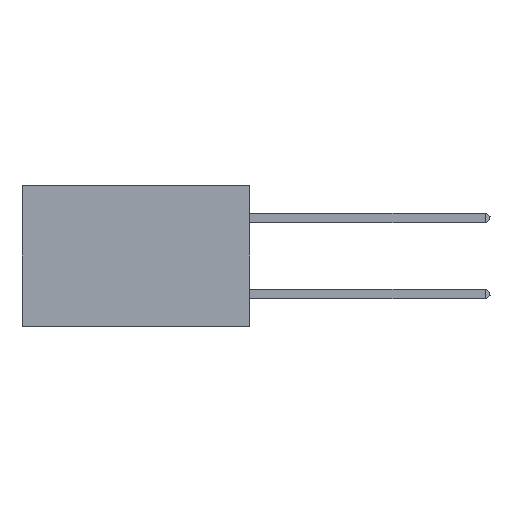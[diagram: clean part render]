
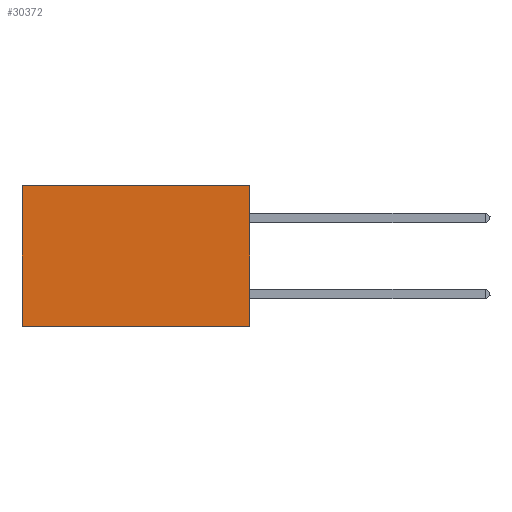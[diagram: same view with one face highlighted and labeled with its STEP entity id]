
A CAD part, left-side view. The second image highlights one B-rep face of the part: STEP entity #30372.
In plain terms, the highlighted planar face has unit normal (-1, 0, 0).
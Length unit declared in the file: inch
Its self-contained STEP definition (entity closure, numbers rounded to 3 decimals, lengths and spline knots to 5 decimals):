
#605 = DIRECTION ( 'NONE',  ( 0., 1., 0. ) ) ;
#3188 = ORIENTED_EDGE ( 'NONE', *, *, #27083, .F. ) ;
#3413 = DIRECTION ( 'NONE',  ( 0., 0., -1. ) ) ;
#5521 = DIRECTION ( 'NONE',  ( 0., 0., -1. ) ) ;
#5573 = ORIENTED_EDGE ( 'NONE', *, *, #12115, .F. ) ;
#7573 = AXIS2_PLACEMENT_3D ( 'NONE', #19884, #30374, #27205 ) ;
#8574 = EDGE_CURVE ( 'NONE', #14365, #45334, #22347, .T. ) ;
#9254 = CARTESIAN_POINT ( 'NONE',  ( 0.2875, 0.6, 0. ) ) ;
#12115 = EDGE_CURVE ( 'NONE', #43734, #46641, #36750, .T. ) ;
#14365 = VERTEX_POINT ( 'NONE', #9254 ) ;
#14827 = CARTESIAN_POINT ( 'NONE',  ( 0.2875, 0., -0.37 ) ) ;
#17012 = LINE ( 'NONE', #34792, #41972 ) ;
#19884 = CARTESIAN_POINT ( 'NONE',  ( 0.2875, 0., 0. ) ) ;
#21505 = EDGE_CURVE ( 'NONE', #43734, #14365, #17012, .T. ) ;
#22347 = LINE ( 'NONE', #27284, #35377 ) ;
#22692 = CARTESIAN_POINT ( 'NONE',  ( 0.2875, 0., -0.37 ) ) ;
#22699 = EDGE_LOOP ( 'NONE', ( #24024, #3188, #5573, #31889 ) ) ;
#23482 = LINE ( 'NONE', #22692, #39367 ) ;
#24024 = ORIENTED_EDGE ( 'NONE', *, *, #8574, .T. ) ;
#27083 = EDGE_CURVE ( 'NONE', #46641, #45334, #23482, .T. ) ;
#27205 = DIRECTION ( 'NONE',  ( 0., 0., -1. ) ) ;
#27284 = CARTESIAN_POINT ( 'NONE',  ( 0.2875, 0.6, 0. ) ) ;
#30372 = ADVANCED_FACE ( 'NONE', ( #33926 ), #34445, .F. ) ;
#30374 = DIRECTION ( 'NONE',  ( 1., 0., 0. ) ) ;
#30517 = CARTESIAN_POINT ( 'NONE',  ( 0.2875, 0., 0. ) ) ;
#31889 = ORIENTED_EDGE ( 'NONE', *, *, #21505, .T. ) ;
#32306 = CARTESIAN_POINT ( 'NONE',  ( 0.2875, 0., 0. ) ) ;
#33334 = VECTOR ( 'NONE', #3413, 39.37008 ) ;
#33926 = FACE_OUTER_BOUND ( 'NONE', #22699, .T. ) ;
#34445 = PLANE ( 'NONE',  #7573 ) ;
#34792 = CARTESIAN_POINT ( 'NONE',  ( 0.2875, 0., 0. ) ) ;
#35377 = VECTOR ( 'NONE', #5521, 39.37008 ) ;
#36750 = LINE ( 'NONE', #32306, #33334 ) ;
#39367 = VECTOR ( 'NONE', #605, 39.37008 ) ;
#41972 = VECTOR ( 'NONE', #45438, 39.37008 ) ;
#43734 = VERTEX_POINT ( 'NONE', #30517 ) ;
#45334 = VERTEX_POINT ( 'NONE', #46346 ) ;
#45438 = DIRECTION ( 'NONE',  ( 0., 1., 0. ) ) ;
#46346 = CARTESIAN_POINT ( 'NONE',  ( 0.2875, 0.6, -0.37 ) ) ;
#46641 = VERTEX_POINT ( 'NONE', #14827 ) ;
